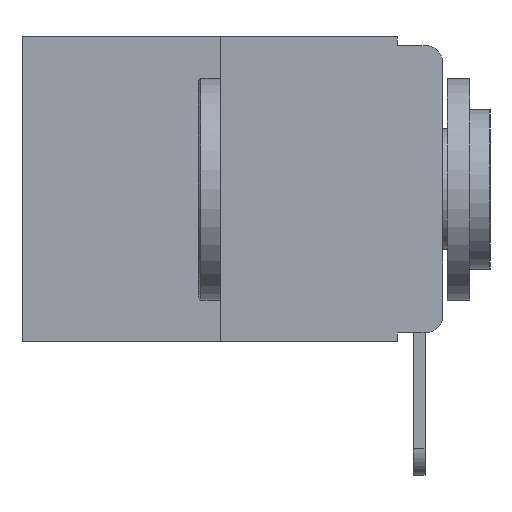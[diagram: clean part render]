
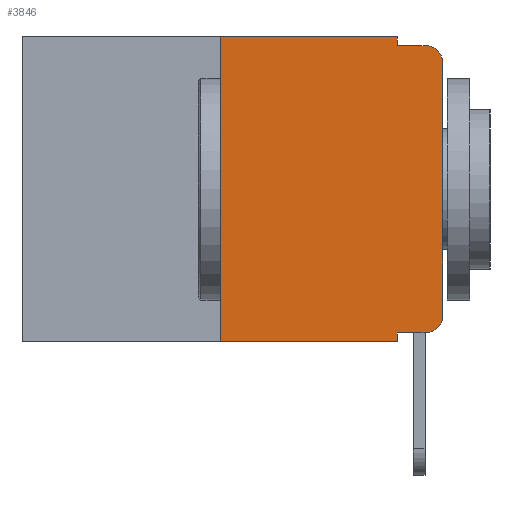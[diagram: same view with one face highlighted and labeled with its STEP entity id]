
A CAD part, left-side view. The second image highlights one B-rep face of the part: STEP entity #3846.
In plain terms, the highlighted planar face has unit normal (-1, 0, 0).
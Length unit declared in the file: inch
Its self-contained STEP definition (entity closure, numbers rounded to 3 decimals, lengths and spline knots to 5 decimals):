
#162 = DIRECTION ( 'NONE',  ( 0., 0., -1. ) ) ;
#270 = VECTOR ( 'NONE', #4899, 39.37008 ) ;
#782 = VERTEX_POINT ( 'NONE', #4142 ) ;
#822 = DIRECTION ( 'NONE',  ( 0., 0., -1. ) ) ;
#1046 = VECTOR ( 'NONE', #17954, 39.37008 ) ;
#1533 = EDGE_CURVE ( 'NONE', #4470, #3966, #2490, .T. ) ;
#1650 = ORIENTED_EDGE ( 'NONE', *, *, #11853, .T. ) ;
#1682 = CARTESIAN_POINT ( 'NONE',  ( 0., 0.051, -0.343 ) ) ;
#2250 = LINE ( 'NONE', #3912, #11159 ) ;
#2380 = EDGE_CURVE ( 'NONE', #3966, #7430, #14118, .T. ) ;
#2490 = LINE ( 'NONE', #8126, #18657 ) ;
#2642 = CARTESIAN_POINT ( 'NONE',  ( 0., 0., -0.03 ) ) ;
#2694 = CARTESIAN_POINT ( 'NONE',  ( 0., 0.25, 0. ) ) ;
#3171 = CIRCLE ( 'NONE', #8188, 0.02 ) ;
#3663 = VECTOR ( 'NONE', #3861, 39.37008 ) ;
#3846 = ADVANCED_FACE ( 'NONE', ( #9453 ), #18475, .F. ) ;
#3861 = DIRECTION ( 'NONE',  ( 0., -1., 0. ) ) ;
#3871 = EDGE_LOOP ( 'NONE', ( #15729, #1650, #7084, #5706, #5462, #5613, #5280, #5125, #4898, #4829 ) ) ;
#3912 = CARTESIAN_POINT ( 'NONE',  ( 0., 0., 0. ) ) ;
#3966 = VERTEX_POINT ( 'NONE', #17449 ) ;
#4142 = CARTESIAN_POINT ( 'NONE',  ( 0., 0.25, -0.343 ) ) ;
#4258 = EDGE_CURVE ( 'NONE', #782, #4688, #13663, .T. ) ;
#4470 = VERTEX_POINT ( 'NONE', #6890 ) ;
#4688 = VERTEX_POINT ( 'NONE', #1682 ) ;
#4829 = ORIENTED_EDGE ( 'NONE', *, *, #19080, .T. ) ;
#4872 = EDGE_CURVE ( 'NONE', #6899, #4688, #10087, .T. ) ;
#4898 = ORIENTED_EDGE ( 'NONE', *, *, #10778, .T. ) ;
#4899 = DIRECTION ( 'NONE',  ( 0., -1., 0. ) ) ;
#5125 = ORIENTED_EDGE ( 'NONE', *, *, #4872, .F. ) ;
#5280 = ORIENTED_EDGE ( 'NONE', *, *, #4258, .T. ) ;
#5462 = ORIENTED_EDGE ( 'NONE', *, *, #6379, .F. ) ;
#5613 = ORIENTED_EDGE ( 'NONE', *, *, #18522, .F. ) ;
#5694 = DIRECTION ( 'NONE',  ( 0., 0., 1. ) ) ;
#5706 = ORIENTED_EDGE ( 'NONE', *, *, #1533, .F. ) ;
#6379 = EDGE_CURVE ( 'NONE', #9233, #4470, #19567, .T. ) ;
#6674 = CIRCLE ( 'NONE', #10068, 0.02 ) ;
#6890 = CARTESIAN_POINT ( 'NONE',  ( 0., 0.051, 0. ) ) ;
#6899 = VERTEX_POINT ( 'NONE', #15290 ) ;
#7084 = ORIENTED_EDGE ( 'NONE', *, *, #2380, .F. ) ;
#7396 = DIRECTION ( 'NONE',  ( -1., 0., 0. ) ) ;
#7430 = VERTEX_POINT ( 'NONE', #20345 ) ;
#8126 = CARTESIAN_POINT ( 'NONE',  ( 0., 0.051, 0. ) ) ;
#8188 = AXIS2_PLACEMENT_3D ( 'NONE', #16429, #7396, #17867 ) ;
#8363 = CARTESIAN_POINT ( 'NONE',  ( 0., 0.051, -0.333 ) ) ;
#8794 = VERTEX_POINT ( 'NONE', #2642 ) ;
#9233 = VERTEX_POINT ( 'NONE', #13471 ) ;
#9453 = FACE_OUTER_BOUND ( 'NONE', #3871, .T. ) ;
#9489 = LINE ( 'NONE', #8363, #270 ) ;
#9735 = DIRECTION ( 'NONE',  ( 1., 0., 0. ) ) ;
#10068 = AXIS2_PLACEMENT_3D ( 'NONE', #19171, #10423, #162 ) ;
#10087 = LINE ( 'NONE', #10873, #13626 ) ;
#10348 = EDGE_CURVE ( 'NONE', #20248, #8794, #2250, .T. ) ;
#10423 = DIRECTION ( 'NONE',  ( -1., 0., 0. ) ) ;
#10778 = EDGE_CURVE ( 'NONE', #6899, #14312, #9489, .T. ) ;
#10873 = CARTESIAN_POINT ( 'NONE',  ( 0., 0.051, 0. ) ) ;
#11159 = VECTOR ( 'NONE', #5694, 39.37008 ) ;
#11853 = EDGE_CURVE ( 'NONE', #8794, #7430, #6674, .T. ) ;
#12182 = AXIS2_PLACEMENT_3D ( 'NONE', #12662, #9735, #19944 ) ;
#12512 = DIRECTION ( 'NONE',  ( 0., -1., 0. ) ) ;
#12662 = CARTESIAN_POINT ( 'NONE',  ( 0., 0.473, 0. ) ) ;
#13176 = VECTOR ( 'NONE', #12512, 39.37008 ) ;
#13471 = CARTESIAN_POINT ( 'NONE',  ( 0., 0.25, 0. ) ) ;
#13529 = CARTESIAN_POINT ( 'NONE',  ( 0., 0.473, 0. ) ) ;
#13626 = VECTOR ( 'NONE', #822, 39.37008 ) ;
#13663 = LINE ( 'NONE', #16902, #13176 ) ;
#14118 = LINE ( 'NONE', #16010, #1046 ) ;
#14312 = VERTEX_POINT ( 'NONE', #14624 ) ;
#14624 = CARTESIAN_POINT ( 'NONE',  ( 0., 0.02, -0.333 ) ) ;
#15290 = CARTESIAN_POINT ( 'NONE',  ( 0., 0.051, -0.333 ) ) ;
#15487 = DIRECTION ( 'NONE',  ( 0., 0., 1. ) ) ;
#15729 = ORIENTED_EDGE ( 'NONE', *, *, #10348, .T. ) ;
#16010 = CARTESIAN_POINT ( 'NONE',  ( 0., 0.051, -0.01 ) ) ;
#16429 = CARTESIAN_POINT ( 'NONE',  ( 0., 0.02, -0.313 ) ) ;
#16902 = CARTESIAN_POINT ( 'NONE',  ( 0., 0.473, -0.343 ) ) ;
#17449 = CARTESIAN_POINT ( 'NONE',  ( 0., 0.051, -0.01 ) ) ;
#17665 = VECTOR ( 'NONE', #15487, 39.37008 ) ;
#17867 = DIRECTION ( 'NONE',  ( 0., 0., -1. ) ) ;
#17954 = DIRECTION ( 'NONE',  ( 0., -1., 0. ) ) ;
#18116 = LINE ( 'NONE', #2694, #17665 ) ;
#18475 = PLANE ( 'NONE',  #12182 ) ;
#18522 = EDGE_CURVE ( 'NONE', #782, #9233, #18116, .T. ) ;
#18624 = DIRECTION ( 'NONE',  ( 0., 0., -1. ) ) ;
#18657 = VECTOR ( 'NONE', #18624, 39.37008 ) ;
#19080 = EDGE_CURVE ( 'NONE', #14312, #20248, #3171, .T. ) ;
#19171 = CARTESIAN_POINT ( 'NONE',  ( 0., 0.02, -0.03 ) ) ;
#19490 = CARTESIAN_POINT ( 'NONE',  ( 0., 0., -0.313 ) ) ;
#19567 = LINE ( 'NONE', #13529, #3663 ) ;
#19944 = DIRECTION ( 'NONE',  ( 0., 0., -1. ) ) ;
#20248 = VERTEX_POINT ( 'NONE', #19490 ) ;
#20345 = CARTESIAN_POINT ( 'NONE',  ( 0., 0.02, -0.01 ) ) ;
